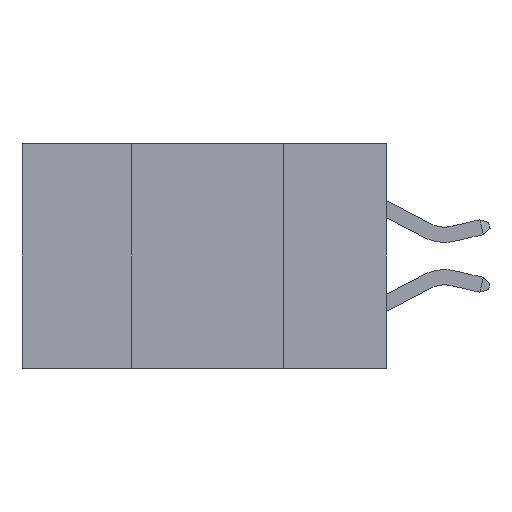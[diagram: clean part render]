
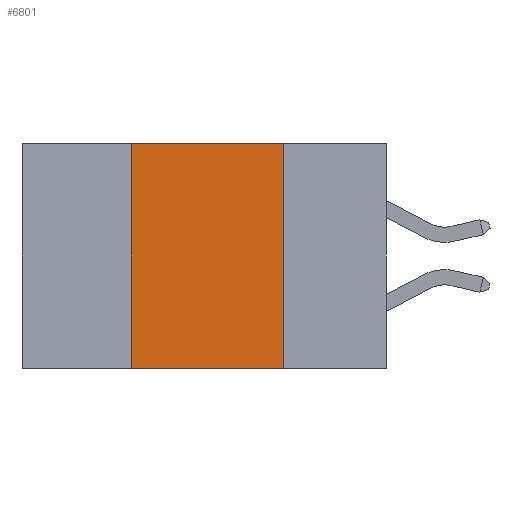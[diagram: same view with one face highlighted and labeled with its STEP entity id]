
A CAD part, left-side view. The second image highlights one B-rep face of the part: STEP entity #6801.
In plain terms, the highlighted planar face has unit normal (-1, 0, 0).
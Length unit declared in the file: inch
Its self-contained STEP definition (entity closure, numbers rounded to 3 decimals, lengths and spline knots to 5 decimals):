
#1220 = DIRECTION ( 'NONE',  ( 0., 0., -1. ) ) ;
#1815 = VECTOR ( 'NONE', #9043, 39.37008 ) ;
#1911 = ORIENTED_EDGE ( 'NONE', *, *, #3377, .F. ) ;
#2533 = DIRECTION ( 'NONE',  ( 1., 0., 0. ) ) ;
#3347 = CARTESIAN_POINT ( 'NONE',  ( 0., 0.42, -0.37 ) ) ;
#3377 = EDGE_CURVE ( 'NONE', #14186, #11735, #14074, .T. ) ;
#3711 = CARTESIAN_POINT ( 'NONE',  ( 0., 0.6, 0. ) ) ;
#4599 = VERTEX_POINT ( 'NONE', #3347 ) ;
#4948 = FACE_OUTER_BOUND ( 'NONE', #16017, .T. ) ;
#5121 = VECTOR ( 'NONE', #8249, 39.37008 ) ;
#5453 = EDGE_CURVE ( 'NONE', #4599, #6664, #14770, .T. ) ;
#5848 = VECTOR ( 'NONE', #8415, 39.37008 ) ;
#6461 = ORIENTED_EDGE ( 'NONE', *, *, #7033, .F. ) ;
#6664 = VERTEX_POINT ( 'NONE', #13204 ) ;
#6801 = ADVANCED_FACE ( 'NONE', ( #4948 ), #15084, .F. ) ;
#7033 = EDGE_CURVE ( 'NONE', #4599, #14186, #14769, .T. ) ;
#8129 = EDGE_CURVE ( 'NONE', #11735, #6664, #10261, .T. ) ;
#8249 = DIRECTION ( 'NONE',  ( 0., 0., 1. ) ) ;
#8415 = DIRECTION ( 'NONE',  ( 0., -1., 0. ) ) ;
#9040 = CARTESIAN_POINT ( 'NONE',  ( 0., 0.42, 0. ) ) ;
#9043 = DIRECTION ( 'NONE',  ( 0., 0., -1. ) ) ;
#10261 = LINE ( 'NONE', #15298, #1815 ) ;
#10262 = CARTESIAN_POINT ( 'NONE',  ( 0., 0.6, 0. ) ) ;
#10364 = ORIENTED_EDGE ( 'NONE', *, *, #8129, .F. ) ;
#10386 = AXIS2_PLACEMENT_3D ( 'NONE', #3711, #2533, #1220 ) ;
#11735 = VERTEX_POINT ( 'NONE', #16226 ) ;
#13204 = CARTESIAN_POINT ( 'NONE',  ( 0., 0.17, -0.37 ) ) ;
#13268 = CARTESIAN_POINT ( 'NONE',  ( 0., 0.6, -0.37 ) ) ;
#14074 = LINE ( 'NONE', #10262, #16127 ) ;
#14186 = VERTEX_POINT ( 'NONE', #9040 ) ;
#14526 = CARTESIAN_POINT ( 'NONE',  ( 0., 0.42, -0.37 ) ) ;
#14769 = LINE ( 'NONE', #14526, #5121 ) ;
#14770 = LINE ( 'NONE', #13268, #5848 ) ;
#14961 = ORIENTED_EDGE ( 'NONE', *, *, #5453, .T. ) ;
#15084 = PLANE ( 'NONE',  #10386 ) ;
#15298 = CARTESIAN_POINT ( 'NONE',  ( 0., 0.17, -0.37 ) ) ;
#15300 = DIRECTION ( 'NONE',  ( 0., -1., 0. ) ) ;
#16017 = EDGE_LOOP ( 'NONE', ( #10364, #1911, #6461, #14961 ) ) ;
#16127 = VECTOR ( 'NONE', #15300, 39.37008 ) ;
#16226 = CARTESIAN_POINT ( 'NONE',  ( 0., 0.17, 0. ) ) ;
